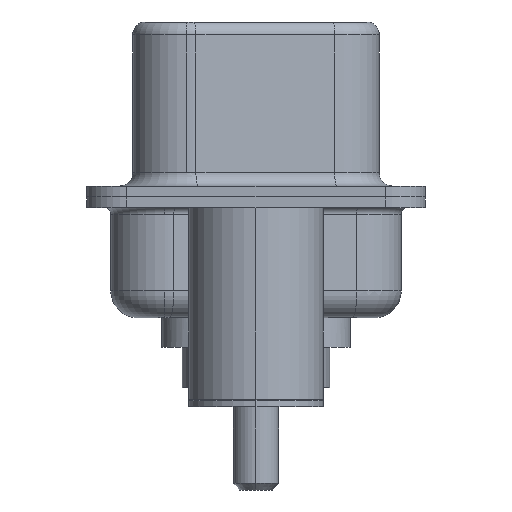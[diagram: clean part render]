
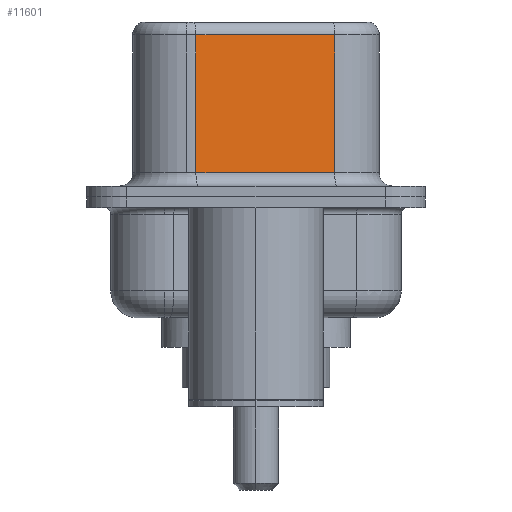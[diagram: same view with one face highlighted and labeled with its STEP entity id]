
A CAD part, left-side view. The second image highlights one B-rep face of the part: STEP entity #11601.
In plain terms, the highlighted planar face has unit normal (-0.985, -0.174, 0).
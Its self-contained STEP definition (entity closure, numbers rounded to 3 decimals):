
#209 = DIRECTION ( 'NONE',  ( 0.174, -0.985, 0. ) ) ;
#758 = VECTOR ( 'NONE', #209, 1000. ) ;
#1391 = CARTESIAN_POINT ( 'NONE',  ( 4.565, -2.927, 6.52 ) ) ;
#1853 = CARTESIAN_POINT ( 'NONE',  ( 4.565, -2.927, 0.9 ) ) ;
#2169 = EDGE_CURVE ( 'NONE', #10634, #2382, #10787, .T. ) ;
#2263 = DIRECTION ( 'NONE',  ( -0.174, 0.985, 0. ) ) ;
#2382 = VERTEX_POINT ( 'NONE', #10414 ) ;
#2703 = DIRECTION ( 'NONE',  ( 0., 0., -1. ) ) ;
#2741 = CARTESIAN_POINT ( 'NONE',  ( 3.655, 2.233, 6.52 ) ) ;
#2794 = ORIENTED_EDGE ( 'NONE', *, *, #2169, .T. ) ;
#3575 = VECTOR ( 'NONE', #7873, 1000. ) ;
#3617 = EDGE_CURVE ( 'NONE', #6411, #8906, #13118, .T. ) ;
#3727 = VECTOR ( 'NONE', #2703, 1000. ) ;
#5324 = CARTESIAN_POINT ( 'NONE',  ( 3.655, 2.233, 0.9 ) ) ;
#5620 = EDGE_CURVE ( 'NONE', #8906, #10634, #13790, .T. ) ;
#6411 = VERTEX_POINT ( 'NONE', #11247 ) ;
#6472 = AXIS2_PLACEMENT_3D ( 'NONE', #7212, #9725, #2263 ) ;
#7212 = CARTESIAN_POINT ( 'NONE',  ( 4.565, -2.927, 6.52 ) ) ;
#7873 = DIRECTION ( 'NONE',  ( -0.174, 0.985, 0. ) ) ;
#8195 = EDGE_LOOP ( 'NONE', ( #11410, #10381, #10528, #2794 ) ) ;
#8906 = VERTEX_POINT ( 'NONE', #10812 ) ;
#9253 = DIRECTION ( 'NONE',  ( 0., 0., -1. ) ) ;
#9303 = VECTOR ( 'NONE', #9253, 1000. ) ;
#9675 = PLANE ( 'NONE',  #6472 ) ;
#9725 = DIRECTION ( 'NONE',  ( 0.985, 0.174, 0. ) ) ;
#10381 = ORIENTED_EDGE ( 'NONE', *, *, #3617, .T. ) ;
#10414 = CARTESIAN_POINT ( 'NONE',  ( 4.565, -2.927, 0.9 ) ) ;
#10528 = ORIENTED_EDGE ( 'NONE', *, *, #5620, .T. ) ;
#10634 = VERTEX_POINT ( 'NONE', #5324 ) ;
#10787 = LINE ( 'NONE', #1853, #758 ) ;
#10812 = CARTESIAN_POINT ( 'NONE',  ( 3.655, 2.233, 6.02 ) ) ;
#11096 = LINE ( 'NONE', #1391, #3727 ) ;
#11247 = CARTESIAN_POINT ( 'NONE',  ( 4.565, -2.927, 6.02 ) ) ;
#11410 = ORIENTED_EDGE ( 'NONE', *, *, #14989, .F. ) ;
#11601 = ADVANCED_FACE ( 'NONE', ( #12748 ), #9675, .F. ) ;
#12173 = CARTESIAN_POINT ( 'NONE',  ( 4.565, -2.927, 6.02 ) ) ;
#12748 = FACE_OUTER_BOUND ( 'NONE', #8195, .T. ) ;
#13118 = LINE ( 'NONE', #12173, #3575 ) ;
#13790 = LINE ( 'NONE', #2741, #9303 ) ;
#14989 = EDGE_CURVE ( 'NONE', #6411, #2382, #11096, .T. ) ;
